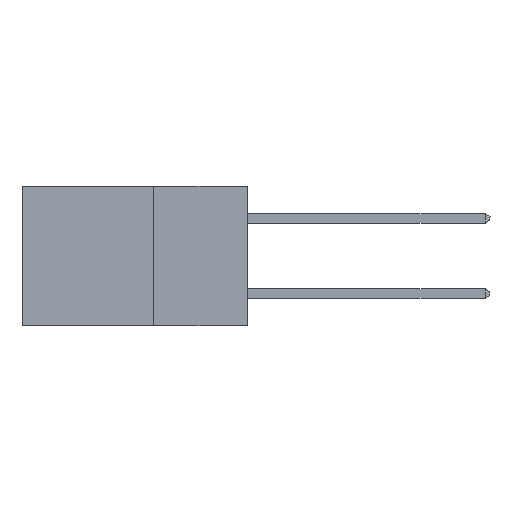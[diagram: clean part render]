
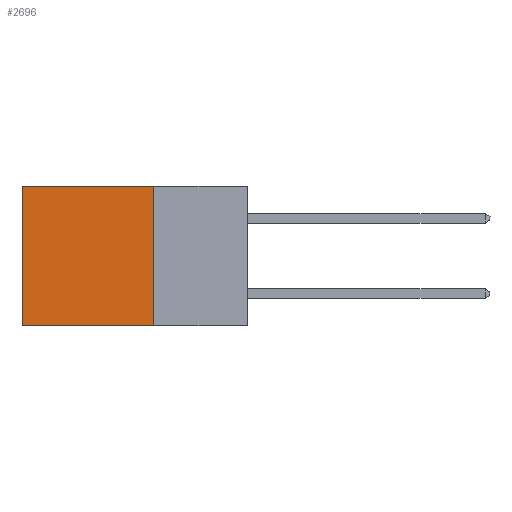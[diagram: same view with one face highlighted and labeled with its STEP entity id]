
A CAD part, left-side view. The second image highlights one B-rep face of the part: STEP entity #2696.
In plain terms, the highlighted planar face has unit normal (-1, 0, 0).
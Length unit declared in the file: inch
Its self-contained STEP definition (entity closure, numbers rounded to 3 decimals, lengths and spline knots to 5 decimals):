
#647 = CARTESIAN_POINT ( 'NONE',  ( 0.2615, 0.6, -0.37 ) ) ;
#684 = CARTESIAN_POINT ( 'NONE',  ( 0.2615, 0.25, 0. ) ) ;
#728 = LINE ( 'NONE', #2785, #7052 ) ;
#874 = EDGE_LOOP ( 'NONE', ( #3344, #985, #1022, #1619 ) ) ;
#985 = ORIENTED_EDGE ( 'NONE', *, *, #8088, .F. ) ;
#996 = VERTEX_POINT ( 'NONE', #684 ) ;
#1022 = ORIENTED_EDGE ( 'NONE', *, *, #5804, .F. ) ;
#1093 = VECTOR ( 'NONE', #8199, 39.37008 ) ;
#1274 = CARTESIAN_POINT ( 'NONE',  ( 0.2615, 0.25, -0.37 ) ) ;
#1619 = ORIENTED_EDGE ( 'NONE', *, *, #5209, .T. ) ;
#1630 = CARTESIAN_POINT ( 'NONE',  ( 0.2615, 0.25, -0.37 ) ) ;
#2696 = ADVANCED_FACE ( 'NONE', ( #9496 ), #2950, .F. ) ;
#2785 = CARTESIAN_POINT ( 'NONE',  ( 0.2615, 0.25, 0. ) ) ;
#2911 = DIRECTION ( 'NONE',  ( 1., 0., 0. ) ) ;
#2950 = PLANE ( 'NONE',  #8619 ) ;
#2980 = DIRECTION ( 'NONE',  ( 0., 1., 0. ) ) ;
#3005 = DIRECTION ( 'NONE',  ( 0., 0., -1. ) ) ;
#3290 = VECTOR ( 'NONE', #4939, 39.37008 ) ;
#3336 = CARTESIAN_POINT ( 'NONE',  ( 0.2615, 0.25, -0.37 ) ) ;
#3344 = ORIENTED_EDGE ( 'NONE', *, *, #7066, .T. ) ;
#3424 = LINE ( 'NONE', #647, #3290 ) ;
#4208 = LINE ( 'NONE', #1274, #5926 ) ;
#4939 = DIRECTION ( 'NONE',  ( 0., 0., -1. ) ) ;
#5198 = CARTESIAN_POINT ( 'NONE',  ( 0.2615, 0.25, -0.37 ) ) ;
#5209 = EDGE_CURVE ( 'NONE', #996, #8913, #728, .T. ) ;
#5578 = DIRECTION ( 'NONE',  ( 0., 1., 0. ) ) ;
#5804 = EDGE_CURVE ( 'NONE', #996, #9108, #8296, .T. ) ;
#5880 = VERTEX_POINT ( 'NONE', #6096 ) ;
#5926 = VECTOR ( 'NONE', #5578, 39.37008 ) ;
#6096 = CARTESIAN_POINT ( 'NONE',  ( 0.2615, 0.6, -0.37 ) ) ;
#7052 = VECTOR ( 'NONE', #2980, 39.37008 ) ;
#7066 = EDGE_CURVE ( 'NONE', #8913, #5880, #3424, .T. ) ;
#8088 = EDGE_CURVE ( 'NONE', #9108, #5880, #4208, .T. ) ;
#8149 = CARTESIAN_POINT ( 'NONE',  ( 0.2615, 0.6, 0. ) ) ;
#8199 = DIRECTION ( 'NONE',  ( 0., 0., -1. ) ) ;
#8296 = LINE ( 'NONE', #1630, #1093 ) ;
#8619 = AXIS2_PLACEMENT_3D ( 'NONE', #5198, #2911, #3005 ) ;
#8913 = VERTEX_POINT ( 'NONE', #8149 ) ;
#9108 = VERTEX_POINT ( 'NONE', #3336 ) ;
#9496 = FACE_OUTER_BOUND ( 'NONE', #874, .T. ) ;
